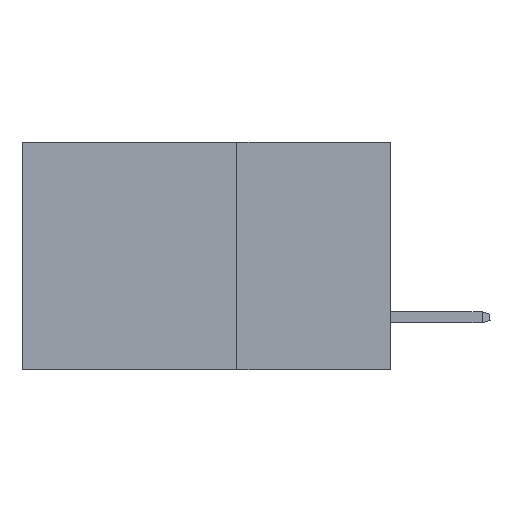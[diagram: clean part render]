
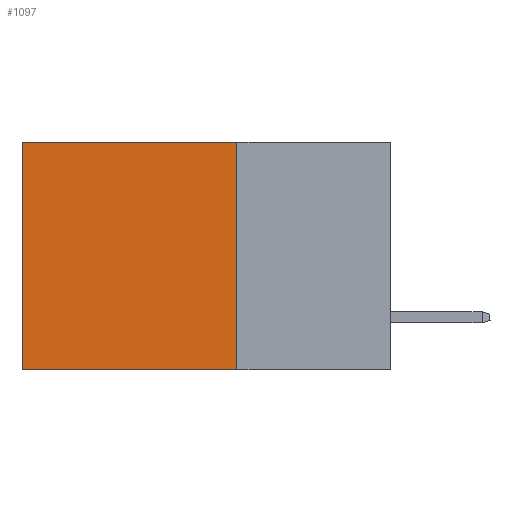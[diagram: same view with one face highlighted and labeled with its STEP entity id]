
A CAD part, left-side view. The second image highlights one B-rep face of the part: STEP entity #1097.
In plain terms, the highlighted planar face has unit normal (-1, 0, 0).
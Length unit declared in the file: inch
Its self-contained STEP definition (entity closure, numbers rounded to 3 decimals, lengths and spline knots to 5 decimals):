
#1097 = ADVANCED_FACE ( 'NONE', ( #9141 ), #16531, .F. ) ;
#1300 = EDGE_CURVE ( 'NONE', #15397, #13337, #2630, .T. ) ;
#2630 = LINE ( 'NONE', #14378, #10557 ) ;
#3418 = CARTESIAN_POINT ( 'NONE',  ( 0.2875, 0.25, -0.37 ) ) ;
#3640 = CARTESIAN_POINT ( 'NONE',  ( 0.2875, 0.25, 0. ) ) ;
#3693 = CARTESIAN_POINT ( 'NONE',  ( 0.2875, 0.25, -0.37 ) ) ;
#3714 = CARTESIAN_POINT ( 'NONE',  ( 0.2875, 0.6, -0.37 ) ) ;
#5039 = VECTOR ( 'NONE', #19304, 39.37008 ) ;
#8349 = EDGE_LOOP ( 'NONE', ( #11685, #12429, #16478, #8838 ) ) ;
#8838 = ORIENTED_EDGE ( 'NONE', *, *, #18649, .T. ) ;
#9141 = FACE_OUTER_BOUND ( 'NONE', #8349, .T. ) ;
#9486 = VECTOR ( 'NONE', #14369, 39.37008 ) ;
#9951 = LINE ( 'NONE', #3640, #9486 ) ;
#10230 = EDGE_CURVE ( 'NONE', #17858, #11982, #9951, .T. ) ;
#10557 = VECTOR ( 'NONE', #12856, 39.37008 ) ;
#10689 = DIRECTION ( 'NONE',  ( 0., 1., 0. ) ) ;
#11450 = LINE ( 'NONE', #13602, #17730 ) ;
#11685 = ORIENTED_EDGE ( 'NONE', *, *, #1300, .T. ) ;
#11982 = VERTEX_POINT ( 'NONE', #3418 ) ;
#12429 = ORIENTED_EDGE ( 'NONE', *, *, #16845, .F. ) ;
#12856 = DIRECTION ( 'NONE',  ( 0., 0., -1. ) ) ;
#13145 = DIRECTION ( 'NONE',  ( 1., 0., 0. ) ) ;
#13220 = CARTESIAN_POINT ( 'NONE',  ( 0.2875, 0.25, 0. ) ) ;
#13337 = VERTEX_POINT ( 'NONE', #3714 ) ;
#13602 = CARTESIAN_POINT ( 'NONE',  ( 0.2875, 0.25, 0. ) ) ;
#13819 = CARTESIAN_POINT ( 'NONE',  ( 0.2875, 0.6, 0. ) ) ;
#14369 = DIRECTION ( 'NONE',  ( 0., 0., -1. ) ) ;
#14378 = CARTESIAN_POINT ( 'NONE',  ( 0.2875, 0.6, 0. ) ) ;
#14684 = DIRECTION ( 'NONE',  ( 0., 0., -1. ) ) ;
#15397 = VERTEX_POINT ( 'NONE', #13819 ) ;
#16002 = CARTESIAN_POINT ( 'NONE',  ( 0.2875, 0.25, 0. ) ) ;
#16478 = ORIENTED_EDGE ( 'NONE', *, *, #10230, .F. ) ;
#16531 = PLANE ( 'NONE',  #19393 ) ;
#16845 = EDGE_CURVE ( 'NONE', #11982, #13337, #19224, .T. ) ;
#17730 = VECTOR ( 'NONE', #10689, 39.37008 ) ;
#17858 = VERTEX_POINT ( 'NONE', #16002 ) ;
#18649 = EDGE_CURVE ( 'NONE', #17858, #15397, #11450, .T. ) ;
#19224 = LINE ( 'NONE', #3693, #5039 ) ;
#19304 = DIRECTION ( 'NONE',  ( 0., 1., 0. ) ) ;
#19393 = AXIS2_PLACEMENT_3D ( 'NONE', #13220, #13145, #14684 ) ;
